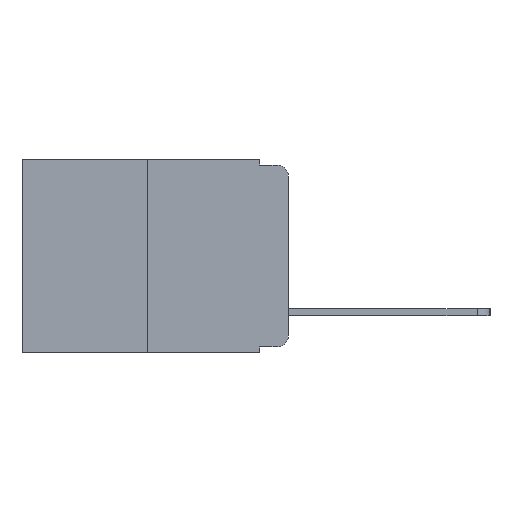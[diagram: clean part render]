
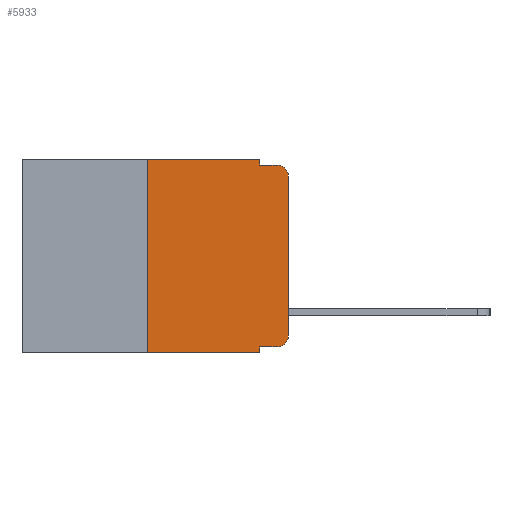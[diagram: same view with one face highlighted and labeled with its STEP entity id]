
A CAD part, left-side view. The second image highlights one B-rep face of the part: STEP entity #5933.
In plain terms, the highlighted planar face has unit normal (-1, 0, 0).
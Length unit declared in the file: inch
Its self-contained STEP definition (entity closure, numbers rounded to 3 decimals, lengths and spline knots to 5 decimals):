
#7 = CARTESIAN_POINT ( 'NONE',  ( 0., 0.051, 0. ) ) ;
#455 = EDGE_CURVE ( 'NONE', #11895, #1294, #4028, .T. ) ;
#873 = VECTOR ( 'NONE', #14125, 39.37008 ) ;
#893 = DIRECTION ( 'NONE',  ( -1., 0., 0. ) ) ;
#1126 = CARTESIAN_POINT ( 'NONE',  ( 0., 0.051, 0. ) ) ;
#1158 = AXIS2_PLACEMENT_3D ( 'NONE', #11634, #16031, #7221 ) ;
#1294 = VERTEX_POINT ( 'NONE', #9543 ) ;
#1461 = EDGE_CURVE ( 'NONE', #4013, #2753, #14084, .T. ) ;
#1469 = CARTESIAN_POINT ( 'NONE',  ( 0., 0.051, -0.343 ) ) ;
#1595 = LINE ( 'NONE', #3033, #17472 ) ;
#1638 = VECTOR ( 'NONE', #13040, 39.37008 ) ;
#1687 = ORIENTED_EDGE ( 'NONE', *, *, #5875, .T. ) ;
#2377 = CARTESIAN_POINT ( 'NONE',  ( 0., 0.051, 0. ) ) ;
#2621 = VERTEX_POINT ( 'NONE', #1469 ) ;
#2753 = VERTEX_POINT ( 'NONE', #3652 ) ;
#2960 = ORIENTED_EDGE ( 'NONE', *, *, #15906, .T. ) ;
#3033 = CARTESIAN_POINT ( 'NONE',  ( 0., 0.051, -0.01 ) ) ;
#3076 = CARTESIAN_POINT ( 'NONE',  ( 0., 0., 0. ) ) ;
#3648 = LINE ( 'NONE', #6850, #18962 ) ;
#3652 = CARTESIAN_POINT ( 'NONE',  ( 0., 0.051, -0.01 ) ) ;
#3781 = DIRECTION ( 'NONE',  ( 0., -1., 0. ) ) ;
#4011 = CARTESIAN_POINT ( 'NONE',  ( 0., 0.051, -0.333 ) ) ;
#4013 = VERTEX_POINT ( 'NONE', #1126 ) ;
#4028 = LINE ( 'NONE', #17337, #8105 ) ;
#4355 = ORIENTED_EDGE ( 'NONE', *, *, #6632, .T. ) ;
#4697 = CIRCLE ( 'NONE', #8569, 0.02 ) ;
#5033 = ORIENTED_EDGE ( 'NONE', *, *, #17828, .F. ) ;
#5062 = CARTESIAN_POINT ( 'NONE',  ( 0., 0., -0.313 ) ) ;
#5464 = VERTEX_POINT ( 'NONE', #10209 ) ;
#5580 = CARTESIAN_POINT ( 'NONE',  ( 0., 0., -0.03 ) ) ;
#5600 = EDGE_CURVE ( 'NONE', #2753, #5464, #1595, .T. ) ;
#5875 = EDGE_CURVE ( 'NONE', #11895, #2621, #12945, .T. ) ;
#5933 = ADVANCED_FACE ( 'NONE', ( #19237 ), #8624, .F. ) ;
#5935 = DIRECTION ( 'NONE',  ( -1., 0., 0. ) ) ;
#6059 = ORIENTED_EDGE ( 'NONE', *, *, #12991, .T. ) ;
#6632 = EDGE_CURVE ( 'NONE', #17031, #5464, #4697, .T. ) ;
#6850 = CARTESIAN_POINT ( 'NONE',  ( 0., 0.473, 0. ) ) ;
#7043 = EDGE_CURVE ( 'NONE', #1294, #4013, #3648, .T. ) ;
#7221 = DIRECTION ( 'NONE',  ( 0., 0., -1. ) ) ;
#7649 = DIRECTION ( 'NONE',  ( 0., 0., -1. ) ) ;
#7716 = ORIENTED_EDGE ( 'NONE', *, *, #7043, .F. ) ;
#8105 = VECTOR ( 'NONE', #17319, 39.37008 ) ;
#8173 = ORIENTED_EDGE ( 'NONE', *, *, #5600, .F. ) ;
#8569 = AXIS2_PLACEMENT_3D ( 'NONE', #14806, #5935, #16263 ) ;
#8611 = EDGE_CURVE ( 'NONE', #11027, #17031, #18688, .T. ) ;
#8624 = PLANE ( 'NONE',  #1158 ) ;
#8721 = CIRCLE ( 'NONE', #10778, 0.02 ) ;
#8757 = CARTESIAN_POINT ( 'NONE',  ( 0., 0.051, -0.333 ) ) ;
#8787 = LINE ( 'NONE', #4011, #1638 ) ;
#8932 = LINE ( 'NONE', #7, #12455 ) ;
#9543 = CARTESIAN_POINT ( 'NONE',  ( 0., 0.25, 0. ) ) ;
#9979 = CARTESIAN_POINT ( 'NONE',  ( 0., 0.02, -0.313 ) ) ;
#10209 = CARTESIAN_POINT ( 'NONE',  ( 0., 0.02, -0.01 ) ) ;
#10778 = AXIS2_PLACEMENT_3D ( 'NONE', #9979, #893, #11487 ) ;
#11027 = VERTEX_POINT ( 'NONE', #5062 ) ;
#11487 = DIRECTION ( 'NONE',  ( 0., 0., -1. ) ) ;
#11634 = CARTESIAN_POINT ( 'NONE',  ( 0., 0.473, 0. ) ) ;
#11895 = VERTEX_POINT ( 'NONE', #18994 ) ;
#12455 = VECTOR ( 'NONE', #7649, 39.37008 ) ;
#12945 = LINE ( 'NONE', #15588, #873 ) ;
#12991 = EDGE_CURVE ( 'NONE', #17979, #11027, #8721, .T. ) ;
#13040 = DIRECTION ( 'NONE',  ( 0., -1., 0. ) ) ;
#13220 = ORIENTED_EDGE ( 'NONE', *, *, #455, .F. ) ;
#13564 = DIRECTION ( 'NONE',  ( 0., -1., 0. ) ) ;
#13638 = VECTOR ( 'NONE', #17332, 39.37008 ) ;
#14084 = LINE ( 'NONE', #2377, #13638 ) ;
#14125 = DIRECTION ( 'NONE',  ( 0., -1., 0. ) ) ;
#14202 = EDGE_LOOP ( 'NONE', ( #17800, #4355, #8173, #16308, #7716, #13220, #1687, #5033, #2960, #6059 ) ) ;
#14806 = CARTESIAN_POINT ( 'NONE',  ( 0., 0.02, -0.03 ) ) ;
#14860 = VECTOR ( 'NONE', #15056, 39.37008 ) ;
#15056 = DIRECTION ( 'NONE',  ( 0., 0., 1. ) ) ;
#15326 = VERTEX_POINT ( 'NONE', #8757 ) ;
#15355 = CARTESIAN_POINT ( 'NONE',  ( 0., 0.02, -0.333 ) ) ;
#15588 = CARTESIAN_POINT ( 'NONE',  ( 0., 0.473, -0.343 ) ) ;
#15906 = EDGE_CURVE ( 'NONE', #15326, #17979, #8787, .T. ) ;
#16031 = DIRECTION ( 'NONE',  ( 1., 0., 0. ) ) ;
#16263 = DIRECTION ( 'NONE',  ( 0., 0., -1. ) ) ;
#16308 = ORIENTED_EDGE ( 'NONE', *, *, #1461, .F. ) ;
#17031 = VERTEX_POINT ( 'NONE', #5580 ) ;
#17319 = DIRECTION ( 'NONE',  ( 0., 0., 1. ) ) ;
#17332 = DIRECTION ( 'NONE',  ( 0., 0., -1. ) ) ;
#17337 = CARTESIAN_POINT ( 'NONE',  ( 0., 0.25, 0. ) ) ;
#17472 = VECTOR ( 'NONE', #13564, 39.37008 ) ;
#17800 = ORIENTED_EDGE ( 'NONE', *, *, #8611, .T. ) ;
#17828 = EDGE_CURVE ( 'NONE', #15326, #2621, #8932, .T. ) ;
#17979 = VERTEX_POINT ( 'NONE', #15355 ) ;
#18688 = LINE ( 'NONE', #3076, #14860 ) ;
#18962 = VECTOR ( 'NONE', #3781, 39.37008 ) ;
#18994 = CARTESIAN_POINT ( 'NONE',  ( 0., 0.25, -0.343 ) ) ;
#19237 = FACE_OUTER_BOUND ( 'NONE', #14202, .T. ) ;
